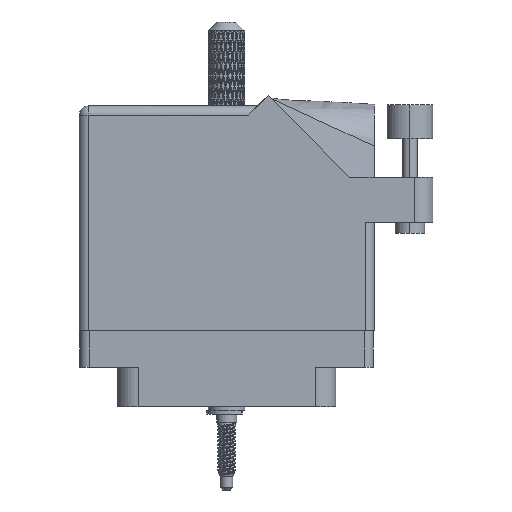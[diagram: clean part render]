
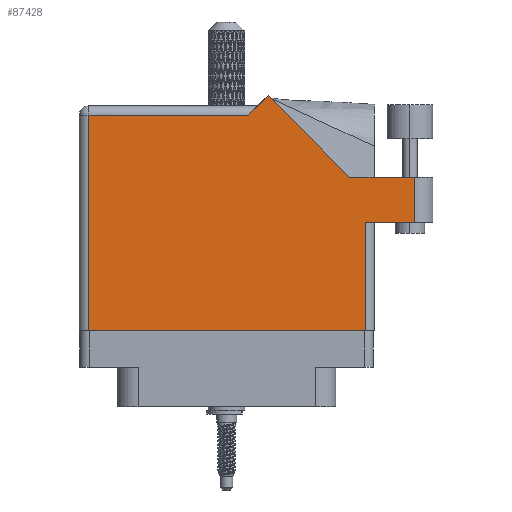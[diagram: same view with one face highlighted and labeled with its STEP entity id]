
A CAD part, front view. The second image highlights one B-rep face of the part: STEP entity #87428.
In plain terms, the highlighted face is planar.
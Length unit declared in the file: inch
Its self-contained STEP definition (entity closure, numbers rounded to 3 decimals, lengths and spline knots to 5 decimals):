
#431 = ORIENTED_EDGE ( 'NONE', *, *, #75483, .T. ) ;
#2203 = CARTESIAN_POINT ( 'NONE',  ( 1.405, 0.944, 0.455 ) ) ;
#2693 = DIRECTION ( 'NONE',  ( -1., 0., 0. ) ) ;
#7486 = VERTEX_POINT ( 'NONE', #37099 ) ;
#8332 = VERTEX_POINT ( 'NONE', #87945 ) ;
#8807 = LINE ( 'NONE', #2203, #102178 ) ;
#9473 = EDGE_LOOP ( 'NONE', ( #431, #105229, #97952, #90882, #51889, #51261, #83715, #9562, #100525 ) ) ;
#9562 = ORIENTED_EDGE ( 'NONE', *, *, #49049, .T. ) ;
#15877 = DIRECTION ( 'NONE',  ( 0., 1., 0. ) ) ;
#17138 = VECTOR ( 'NONE', #63332, 39.37008 ) ;
#18476 = VECTOR ( 'NONE', #18821, 39.37008 ) ;
#18574 = CARTESIAN_POINT ( 'NONE',  ( -1.005, -0.1, 0.455 ) ) ;
#18821 = DIRECTION ( 'NONE',  ( -1., 0., 0. ) ) ;
#19527 = VECTOR ( 'NONE', #82288, 39.37008 ) ;
#20198 = VECTOR ( 'NONE', #33696, 39.37008 ) ;
#20209 = PLANE ( 'NONE',  #83697 ) ;
#21139 = DIRECTION ( 'NONE',  ( -1., 0., 0. ) ) ;
#24592 = CARTESIAN_POINT ( 'NONE',  ( 0.83942, 0.944, 0.455 ) ) ;
#28395 = CARTESIAN_POINT ( 'NONE',  ( -1.005, 1.43, 0.455 ) ) ;
#32469 = LINE ( 'NONE', #92133, #18476 ) ;
#33121 = EDGE_CURVE ( 'NONE', #100001, #8332, #57366, .T. ) ;
#33279 = CARTESIAN_POINT ( 'NONE',  ( 1.28, 0.944, 0.455 ) ) ;
#33696 = DIRECTION ( 'NONE',  ( 1., 0., 0. ) ) ;
#34952 = CARTESIAN_POINT ( 'NONE',  ( 1.28, 0.637, 0.455 ) ) ;
#34997 = CARTESIAN_POINT ( 'NONE',  ( -0.943, -0.1, 0.455 ) ) ;
#36543 = DIRECTION ( 'NONE',  ( 0., 0., -1. ) ) ;
#37099 = CARTESIAN_POINT ( 'NONE',  ( -0.943, 1.368, 0.455 ) ) ;
#37757 = LINE ( 'NONE', #44808, #42905 ) ;
#38296 = VERTEX_POINT ( 'NONE', #34997 ) ;
#39703 = VERTEX_POINT ( 'NONE', #87229 ) ;
#41437 = CARTESIAN_POINT ( 'NONE',  ( 0.212, 1.43, 0.455 ) ) ;
#41633 = DIRECTION ( 'NONE',  ( -0.707, 0.707, 0. ) ) ;
#41873 = EDGE_CURVE ( 'NONE', #72630, #100001, #8807, .T. ) ;
#42711 = EDGE_CURVE ( 'NONE', #72470, #72630, #105832, .T. ) ;
#42905 = VECTOR ( 'NONE', #53400, 39.37008 ) ;
#44808 = CARTESIAN_POINT ( 'NONE',  ( 0.943, 0.637, 0.455 ) ) ;
#44964 = VECTOR ( 'NONE', #51035, 39.37008 ) ;
#47052 = EDGE_CURVE ( 'NONE', #7486, #38296, #69521, .T. ) ;
#47551 = LINE ( 'NONE', #18574, #44964 ) ;
#49049 = EDGE_CURVE ( 'NONE', #38296, #52698, #47551, .T. ) ;
#50798 = VECTOR ( 'NONE', #15877, 39.37008 ) ;
#51035 = DIRECTION ( 'NONE',  ( 1., 0., 0. ) ) ;
#51261 = ORIENTED_EDGE ( 'NONE', *, *, #65926, .T. ) ;
#51889 = ORIENTED_EDGE ( 'NONE', *, *, #99753, .T. ) ;
#52454 = CARTESIAN_POINT ( 'NONE',  ( 1.28, 0.944, 0.455 ) ) ;
#52698 = VERTEX_POINT ( 'NONE', #70740 ) ;
#53400 = DIRECTION ( 'NONE',  ( 0., 1., 0. ) ) ;
#57244 = LINE ( 'NONE', #91018, #20198 ) ;
#57366 = LINE ( 'NONE', #57752, #72669 ) ;
#57730 = EDGE_CURVE ( 'NONE', #52698, #59483, #37757, .T. ) ;
#57752 = CARTESIAN_POINT ( 'NONE',  ( 0.83942, 0.944, 0.455 ) ) ;
#59483 = VERTEX_POINT ( 'NONE', #61191 ) ;
#61191 = CARTESIAN_POINT ( 'NONE',  ( 0.943, 0.637, 0.455 ) ) ;
#63332 = DIRECTION ( 'NONE',  ( 0., -1., 0. ) ) ;
#65926 = EDGE_CURVE ( 'NONE', #39703, #7486, #32469, .T. ) ;
#69521 = LINE ( 'NONE', #71164, #17138 ) ;
#70740 = CARTESIAN_POINT ( 'NONE',  ( 0.943, -0.1, 0.455 ) ) ;
#71164 = CARTESIAN_POINT ( 'NONE',  ( -0.943, -0.1, 0.455 ) ) ;
#72470 = VERTEX_POINT ( 'NONE', #34952 ) ;
#72630 = VERTEX_POINT ( 'NONE', #52454 ) ;
#72669 = VECTOR ( 'NONE', #41633, 39.37008 ) ;
#74476 = LINE ( 'NONE', #41437, #19527 ) ;
#75483 = EDGE_CURVE ( 'NONE', #59483, #72470, #57244, .T. ) ;
#82288 = DIRECTION ( 'NONE',  ( -0.707, -0.707, 0. ) ) ;
#83697 = AXIS2_PLACEMENT_3D ( 'NONE', #28395, #36543, #2693 ) ;
#83715 = ORIENTED_EDGE ( 'NONE', *, *, #47052, .T. ) ;
#87229 = CARTESIAN_POINT ( 'NONE',  ( 0.15, 1.368, 0.455 ) ) ;
#87428 = ADVANCED_FACE ( 'NONE', ( #103654 ), #20209, .F. ) ;
#87945 = CARTESIAN_POINT ( 'NONE',  ( 0.28271, 1.50071, 0.455 ) ) ;
#90882 = ORIENTED_EDGE ( 'NONE', *, *, #33121, .T. ) ;
#91018 = CARTESIAN_POINT ( 'NONE',  ( 1.005, 0.637, 0.455 ) ) ;
#92133 = CARTESIAN_POINT ( 'NONE',  ( -1.005, 1.368, 0.455 ) ) ;
#97952 = ORIENTED_EDGE ( 'NONE', *, *, #41873, .T. ) ;
#99753 = EDGE_CURVE ( 'NONE', #8332, #39703, #74476, .T. ) ;
#100001 = VERTEX_POINT ( 'NONE', #24592 ) ;
#100525 = ORIENTED_EDGE ( 'NONE', *, *, #57730, .T. ) ;
#102178 = VECTOR ( 'NONE', #21139, 39.37008 ) ;
#103654 = FACE_OUTER_BOUND ( 'NONE', #9473, .T. ) ;
#105229 = ORIENTED_EDGE ( 'NONE', *, *, #42711, .T. ) ;
#105832 = LINE ( 'NONE', #33279, #50798 ) ;
